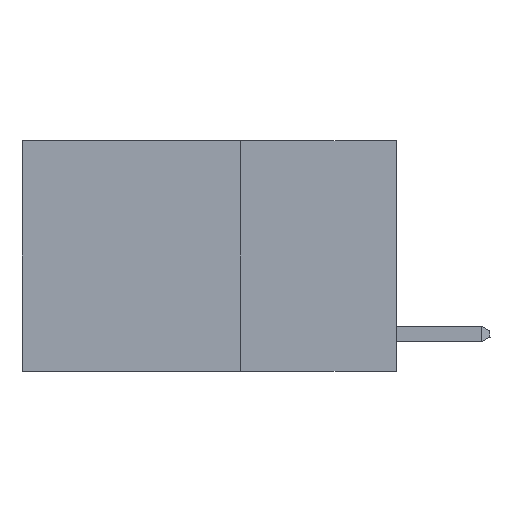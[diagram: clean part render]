
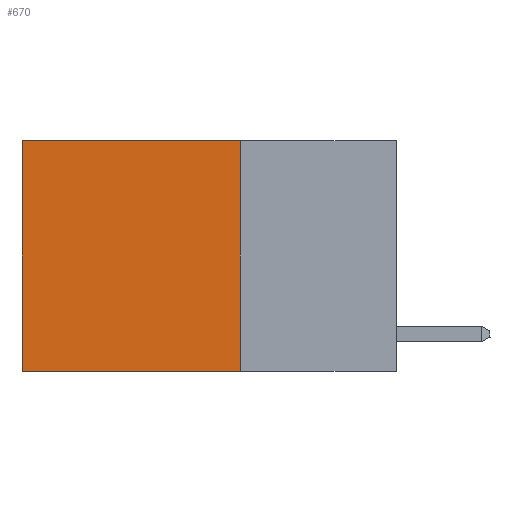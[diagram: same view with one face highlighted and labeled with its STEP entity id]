
A CAD part, left-side view. The second image highlights one B-rep face of the part: STEP entity #670.
In plain terms, the highlighted planar face has unit normal (-1, 0, 0).
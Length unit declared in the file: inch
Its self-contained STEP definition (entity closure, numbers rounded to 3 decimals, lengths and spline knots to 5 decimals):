
#81 = EDGE_LOOP ( 'NONE', ( #17533, #1835, #21775, #1785 ) ) ;
#150 = LINE ( 'NONE', #18841, #17885 ) ;
#411 = VECTOR ( 'NONE', #20756, 39.37008 ) ;
#670 = ADVANCED_FACE ( 'NONE', ( #22710 ), #20745, .F. ) ;
#1785 = ORIENTED_EDGE ( 'NONE', *, *, #11727, .T. ) ;
#1835 = ORIENTED_EDGE ( 'NONE', *, *, #9230, .F. ) ;
#2065 = CARTESIAN_POINT ( 'NONE',  ( 0.2625, 0.25, -0.37 ) ) ;
#2693 = VERTEX_POINT ( 'NONE', #5351 ) ;
#4337 = DIRECTION ( 'NONE',  ( 0., 0., -1. ) ) ;
#4788 = DIRECTION ( 'NONE',  ( 0., 0., -1. ) ) ;
#4813 = LINE ( 'NONE', #20250, #5392 ) ;
#5081 = DIRECTION ( 'NONE',  ( 0., 1., 0. ) ) ;
#5247 = AXIS2_PLACEMENT_3D ( 'NONE', #10235, #22494, #12020 ) ;
#5351 = CARTESIAN_POINT ( 'NONE',  ( 0.2625, 0.6, 0. ) ) ;
#5392 = VECTOR ( 'NONE', #4337, 39.37008 ) ;
#5407 = VECTOR ( 'NONE', #5081, 39.37008 ) ;
#5973 = LINE ( 'NONE', #12180, #5407 ) ;
#6665 = CARTESIAN_POINT ( 'NONE',  ( 0.2625, 0.25, 0. ) ) ;
#8415 = EDGE_CURVE ( 'NONE', #14865, #19996, #150, .T. ) ;
#9230 = EDGE_CURVE ( 'NONE', #19996, #22584, #5973, .T. ) ;
#10235 = CARTESIAN_POINT ( 'NONE',  ( 0.2625, 0.25, 0. ) ) ;
#11727 = EDGE_CURVE ( 'NONE', #14865, #2693, #14607, .T. ) ;
#12020 = DIRECTION ( 'NONE',  ( 0., 0., -1. ) ) ;
#12180 = CARTESIAN_POINT ( 'NONE',  ( 0.2625, 0.25, -0.37 ) ) ;
#12407 = CARTESIAN_POINT ( 'NONE',  ( 0.2625, 0.6, -0.37 ) ) ;
#12832 = EDGE_CURVE ( 'NONE', #2693, #22584, #4813, .T. ) ;
#14522 = CARTESIAN_POINT ( 'NONE',  ( 0.2625, 0.25, 0. ) ) ;
#14607 = LINE ( 'NONE', #6665, #411 ) ;
#14865 = VERTEX_POINT ( 'NONE', #14522 ) ;
#17533 = ORIENTED_EDGE ( 'NONE', *, *, #12832, .T. ) ;
#17885 = VECTOR ( 'NONE', #4788, 39.37008 ) ;
#18841 = CARTESIAN_POINT ( 'NONE',  ( 0.2625, 0.25, 0. ) ) ;
#19996 = VERTEX_POINT ( 'NONE', #2065 ) ;
#20250 = CARTESIAN_POINT ( 'NONE',  ( 0.2625, 0.6, 0. ) ) ;
#20745 = PLANE ( 'NONE',  #5247 ) ;
#20756 = DIRECTION ( 'NONE',  ( 0., 1., 0. ) ) ;
#21775 = ORIENTED_EDGE ( 'NONE', *, *, #8415, .F. ) ;
#22494 = DIRECTION ( 'NONE',  ( 1., 0., 0. ) ) ;
#22584 = VERTEX_POINT ( 'NONE', #12407 ) ;
#22710 = FACE_OUTER_BOUND ( 'NONE', #81, .T. ) ;
